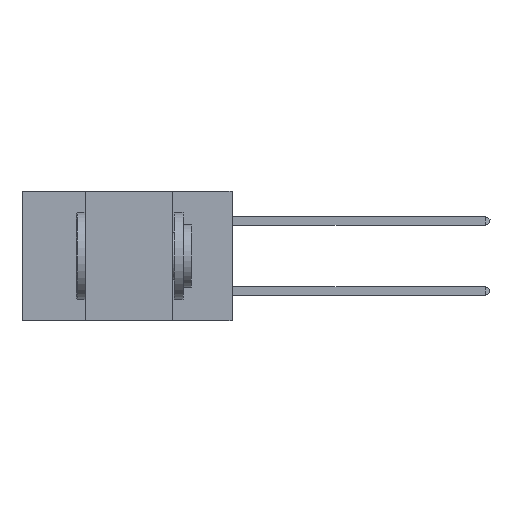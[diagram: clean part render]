
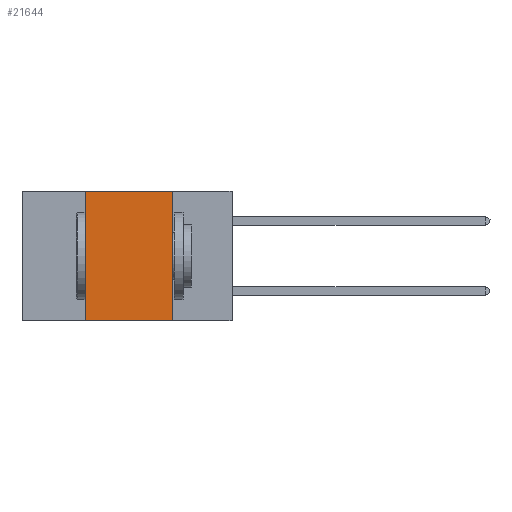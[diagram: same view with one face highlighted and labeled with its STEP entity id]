
A CAD part, left-side view. The second image highlights one B-rep face of the part: STEP entity #21644.
In plain terms, the highlighted planar face has unit normal (-1, 0, 0).
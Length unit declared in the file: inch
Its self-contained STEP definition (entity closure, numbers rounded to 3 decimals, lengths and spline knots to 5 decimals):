
#22 = EDGE_CURVE ( 'NONE', #422, #25256, #33749, .T. ) ;
#422 = VERTEX_POINT ( 'NONE', #10488 ) ;
#560 = VERTEX_POINT ( 'NONE', #35689 ) ;
#608 = CARTESIAN_POINT ( 'NONE',  ( 0., 0.6, 0. ) ) ;
#2604 = CARTESIAN_POINT ( 'NONE',  ( 0., 0.42, 0. ) ) ;
#3431 = CARTESIAN_POINT ( 'NONE',  ( 0., 0.17, 0. ) ) ;
#3506 = LINE ( 'NONE', #2604, #8718 ) ;
#5489 = DIRECTION ( 'NONE',  ( 0., 0., 1. ) ) ;
#5550 = VECTOR ( 'NONE', #6218, 39.37008 ) ;
#6218 = DIRECTION ( 'NONE',  ( 0., 0., -1. ) ) ;
#8718 = VECTOR ( 'NONE', #5489, 39.37008 ) ;
#9469 = CARTESIAN_POINT ( 'NONE',  ( 0., 0.6, 0. ) ) ;
#10488 = CARTESIAN_POINT ( 'NONE',  ( 0., 0.42, -0.37 ) ) ;
#12235 = VECTOR ( 'NONE', #31461, 39.37008 ) ;
#12688 = LINE ( 'NONE', #3431, #5550 ) ;
#14511 = CARTESIAN_POINT ( 'NONE',  ( 0., 0.6, -0.37 ) ) ;
#14991 = FACE_OUTER_BOUND ( 'NONE', #17954, .T. ) ;
#17667 = CARTESIAN_POINT ( 'NONE',  ( 0., 0.17, 0. ) ) ;
#17954 = EDGE_LOOP ( 'NONE', ( #37977, #34142, #20574, #30028 ) ) ;
#18818 = PLANE ( 'NONE',  #31962 ) ;
#18988 = CARTESIAN_POINT ( 'NONE',  ( 0., 0.17, -0.37 ) ) ;
#20574 = ORIENTED_EDGE ( 'NONE', *, *, #28793, .F. ) ;
#21644 = ADVANCED_FACE ( 'NONE', ( #14991 ), #18818, .F. ) ;
#21871 = DIRECTION ( 'NONE',  ( 0., -1., 0. ) ) ;
#25256 = VERTEX_POINT ( 'NONE', #18988 ) ;
#28793 = EDGE_CURVE ( 'NONE', #422, #560, #3506, .T. ) ;
#29505 = LINE ( 'NONE', #9469, #30457 ) ;
#30028 = ORIENTED_EDGE ( 'NONE', *, *, #22, .T. ) ;
#30457 = VECTOR ( 'NONE', #21871, 39.37008 ) ;
#31461 = DIRECTION ( 'NONE',  ( 0., -1., 0. ) ) ;
#31962 = AXIS2_PLACEMENT_3D ( 'NONE', #608, #36955, #34310 ) ;
#32519 = EDGE_CURVE ( 'NONE', #560, #38840, #29505, .T. ) ;
#33749 = LINE ( 'NONE', #14511, #12235 ) ;
#34142 = ORIENTED_EDGE ( 'NONE', *, *, #32519, .F. ) ;
#34310 = DIRECTION ( 'NONE',  ( 0., 0., -1. ) ) ;
#35689 = CARTESIAN_POINT ( 'NONE',  ( 0., 0.42, 0. ) ) ;
#36399 = EDGE_CURVE ( 'NONE', #38840, #25256, #12688, .T. ) ;
#36955 = DIRECTION ( 'NONE',  ( 1., 0., 0. ) ) ;
#37977 = ORIENTED_EDGE ( 'NONE', *, *, #36399, .F. ) ;
#38840 = VERTEX_POINT ( 'NONE', #17667 ) ;
